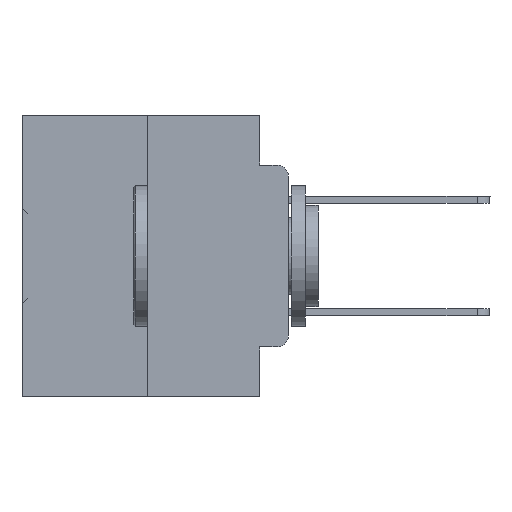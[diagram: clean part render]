
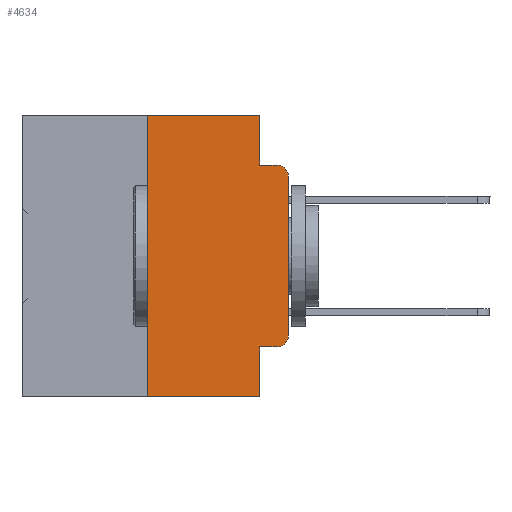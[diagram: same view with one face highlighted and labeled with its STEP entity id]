
A CAD part, left-side view. The second image highlights one B-rep face of the part: STEP entity #4634.
In plain terms, the highlighted planar face has unit normal (-1, 0, 0).
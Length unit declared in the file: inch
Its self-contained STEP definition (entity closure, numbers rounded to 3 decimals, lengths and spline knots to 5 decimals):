
#130 = CARTESIAN_POINT ( 'NONE',  ( 0., 0., -0.3915 ) ) ;
#566 = DIRECTION ( 'NONE',  ( 0., -1., 0. ) ) ;
#579 = EDGE_CURVE ( 'NONE', #6345, #5498, #37587, .T. ) ;
#702 = CARTESIAN_POINT ( 'NONE',  ( 0., 0.051, -0.0885 ) ) ;
#738 = LINE ( 'NONE', #12859, #11951 ) ;
#1114 = ORIENTED_EDGE ( 'NONE', *, *, #31714, .F. ) ;
#1196 = ORIENTED_EDGE ( 'NONE', *, *, #13419, .T. ) ;
#1198 = CARTESIAN_POINT ( 'NONE',  ( 0., 0.051, 0. ) ) ;
#1911 = VECTOR ( 'NONE', #10113, 39.37008 ) ;
#2441 = ORIENTED_EDGE ( 'NONE', *, *, #10100, .T. ) ;
#2491 = VERTEX_POINT ( 'NONE', #37145 ) ;
#3116 = ORIENTED_EDGE ( 'NONE', *, *, #14488, .T. ) ;
#3549 = LINE ( 'NONE', #30920, #1911 ) ;
#4634 = ADVANCED_FACE ( 'NONE', ( #12696 ), #27392, .F. ) ;
#5227 = DIRECTION ( 'NONE',  ( 0., -1., 0. ) ) ;
#5498 = VERTEX_POINT ( 'NONE', #24424 ) ;
#5679 = CIRCLE ( 'NONE', #13252, 0.02 ) ;
#6319 = DIRECTION ( 'NONE',  ( 0., 0., 1. ) ) ;
#6345 = VERTEX_POINT ( 'NONE', #39129 ) ;
#7642 = CARTESIAN_POINT ( 'NONE',  ( 0., 0.25, 0. ) ) ;
#7678 = EDGE_CURVE ( 'NONE', #8208, #11887, #11271, .T. ) ;
#7775 = DIRECTION ( 'NONE',  ( 0., 0., -1. ) ) ;
#8208 = VERTEX_POINT ( 'NONE', #1198 ) ;
#8448 = VERTEX_POINT ( 'NONE', #35316 ) ;
#8491 = CARTESIAN_POINT ( 'NONE',  ( 0., 0.051, 0. ) ) ;
#9160 = DIRECTION ( 'NONE',  ( 1., 0., 0. ) ) ;
#9535 = CIRCLE ( 'NONE', #24722, 0.02 ) ;
#10100 = EDGE_CURVE ( 'NONE', #14703, #32372, #738, .T. ) ;
#10113 = DIRECTION ( 'NONE',  ( 0., -1., 0. ) ) ;
#10849 = DIRECTION ( 'NONE',  ( 0., 0., -1. ) ) ;
#10906 = EDGE_LOOP ( 'NONE', ( #2441, #24147, #16299, #13607, #25155, #29030, #3116, #1114, #15086, #1196 ) ) ;
#11271 = LINE ( 'NONE', #8491, #23333 ) ;
#11887 = VERTEX_POINT ( 'NONE', #702 ) ;
#11951 = VECTOR ( 'NONE', #6319, 39.37008 ) ;
#12696 = FACE_OUTER_BOUND ( 'NONE', #10906, .T. ) ;
#12859 = CARTESIAN_POINT ( 'NONE',  ( 0., 0., 0. ) ) ;
#13252 = AXIS2_PLACEMENT_3D ( 'NONE', #21017, #30123, #29929 ) ;
#13419 = EDGE_CURVE ( 'NONE', #2491, #14703, #9535, .T. ) ;
#13607 = ORIENTED_EDGE ( 'NONE', *, *, #7678, .F. ) ;
#14488 = EDGE_CURVE ( 'NONE', #6345, #8448, #3549, .T. ) ;
#14511 = EDGE_CURVE ( 'NONE', #5498, #8208, #37655, .T. ) ;
#14703 = VERTEX_POINT ( 'NONE', #130 ) ;
#15086 = ORIENTED_EDGE ( 'NONE', *, *, #30685, .T. ) ;
#15430 = VECTOR ( 'NONE', #37778, 39.37008 ) ;
#16299 = ORIENTED_EDGE ( 'NONE', *, *, #34283, .F. ) ;
#16496 = VECTOR ( 'NONE', #566, 39.37008 ) ;
#17037 = VECTOR ( 'NONE', #17305, 39.37008 ) ;
#17305 = DIRECTION ( 'NONE',  ( 0., -1., 0. ) ) ;
#17409 = DIRECTION ( 'NONE',  ( 0., 0., -1. ) ) ;
#17519 = LINE ( 'NONE', #32392, #21953 ) ;
#18142 = VERTEX_POINT ( 'NONE', #26995 ) ;
#19567 = DIRECTION ( 'NONE',  ( -1., 0., 0. ) ) ;
#21017 = CARTESIAN_POINT ( 'NONE',  ( 0., 0.02, -0.1085 ) ) ;
#21953 = VECTOR ( 'NONE', #5227, 39.37008 ) ;
#23333 = VECTOR ( 'NONE', #17409, 39.37008 ) ;
#23472 = CARTESIAN_POINT ( 'NONE',  ( 0., 0.051, -0.0885 ) ) ;
#24147 = ORIENTED_EDGE ( 'NONE', *, *, #34847, .T. ) ;
#24424 = CARTESIAN_POINT ( 'NONE',  ( 0., 0.25, 0. ) ) ;
#24722 = AXIS2_PLACEMENT_3D ( 'NONE', #37197, #19567, #10849 ) ;
#24991 = DIRECTION ( 'NONE',  ( 0., 0., -1. ) ) ;
#25155 = ORIENTED_EDGE ( 'NONE', *, *, #14511, .F. ) ;
#26630 = LINE ( 'NONE', #23472, #17037 ) ;
#26995 = CARTESIAN_POINT ( 'NONE',  ( 0., 0.02, -0.0885 ) ) ;
#27392 = PLANE ( 'NONE',  #29283 ) ;
#27580 = CARTESIAN_POINT ( 'NONE',  ( 0., 0.473, 0. ) ) ;
#27756 = CARTESIAN_POINT ( 'NONE',  ( 0., 0.473, 0. ) ) ;
#28796 = CARTESIAN_POINT ( 'NONE',  ( 0., 0.051, 0. ) ) ;
#28992 = LINE ( 'NONE', #28796, #29626 ) ;
#29030 = ORIENTED_EDGE ( 'NONE', *, *, #579, .F. ) ;
#29283 = AXIS2_PLACEMENT_3D ( 'NONE', #27580, #9160, #24991 ) ;
#29626 = VECTOR ( 'NONE', #7775, 39.37008 ) ;
#29864 = CARTESIAN_POINT ( 'NONE',  ( 0., 0.051, -0.4115 ) ) ;
#29929 = DIRECTION ( 'NONE',  ( 0., 0., -1. ) ) ;
#30123 = DIRECTION ( 'NONE',  ( -1., 0., 0. ) ) ;
#30685 = EDGE_CURVE ( 'NONE', #31011, #2491, #17519, .T. ) ;
#30920 = CARTESIAN_POINT ( 'NONE',  ( 0., 0.473, -0.5 ) ) ;
#31011 = VERTEX_POINT ( 'NONE', #29864 ) ;
#31714 = EDGE_CURVE ( 'NONE', #31011, #8448, #28992, .T. ) ;
#32372 = VERTEX_POINT ( 'NONE', #37363 ) ;
#32392 = CARTESIAN_POINT ( 'NONE',  ( 0., 0.051, -0.4115 ) ) ;
#34283 = EDGE_CURVE ( 'NONE', #11887, #18142, #26630, .T. ) ;
#34847 = EDGE_CURVE ( 'NONE', #32372, #18142, #5679, .T. ) ;
#35316 = CARTESIAN_POINT ( 'NONE',  ( 0., 0.051, -0.5 ) ) ;
#37145 = CARTESIAN_POINT ( 'NONE',  ( 0., 0.02, -0.4115 ) ) ;
#37197 = CARTESIAN_POINT ( 'NONE',  ( 0., 0.02, -0.3915 ) ) ;
#37363 = CARTESIAN_POINT ( 'NONE',  ( 0., 0., -0.1085 ) ) ;
#37587 = LINE ( 'NONE', #7642, #15430 ) ;
#37655 = LINE ( 'NONE', #27756, #16496 ) ;
#37778 = DIRECTION ( 'NONE',  ( 0., 0., 1. ) ) ;
#39129 = CARTESIAN_POINT ( 'NONE',  ( 0., 0.25, -0.5 ) ) ;
